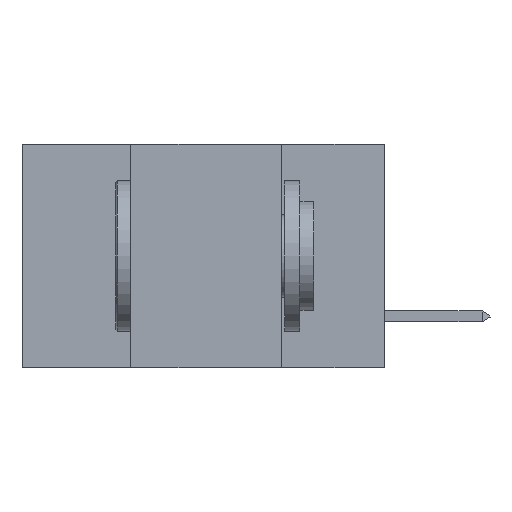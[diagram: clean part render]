
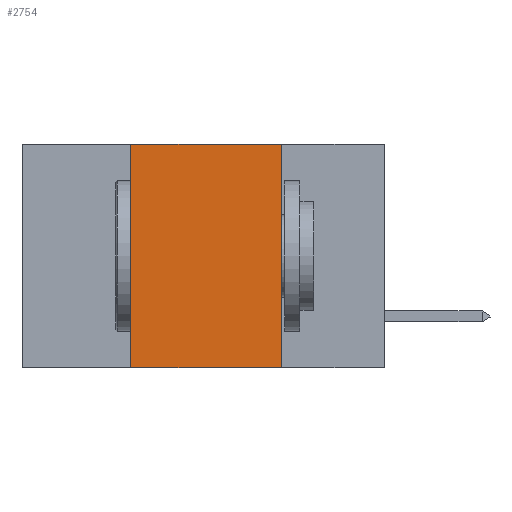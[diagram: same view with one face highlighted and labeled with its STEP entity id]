
A CAD part, left-side view. The second image highlights one B-rep face of the part: STEP entity #2754.
In plain terms, the highlighted planar face has unit normal (-1, 0, 0).
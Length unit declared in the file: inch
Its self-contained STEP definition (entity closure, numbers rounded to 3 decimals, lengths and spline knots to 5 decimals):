
#2 = DIRECTION ( 'NONE',  ( 0., -1., 0. ) ) ;
#82 = DIRECTION ( 'NONE',  ( 0., 0., -1. ) ) ;
#1514 = ORIENTED_EDGE ( 'NONE', *, *, #36094, .F. ) ;
#1586 = VECTOR ( 'NONE', #29866, 39.37008 ) ;
#2420 = VERTEX_POINT ( 'NONE', #3153 ) ;
#2754 = ADVANCED_FACE ( 'NONE', ( #8041 ), #21342, .F. ) ;
#2770 = ORIENTED_EDGE ( 'NONE', *, *, #24472, .F. ) ;
#3153 = CARTESIAN_POINT ( 'NONE',  ( 0., 0.17, -0.37 ) ) ;
#4277 = CARTESIAN_POINT ( 'NONE',  ( 0., 0.17, 0. ) ) ;
#5405 = EDGE_LOOP ( 'NONE', ( #2770, #1514, #38943, #5485 ) ) ;
#5485 = ORIENTED_EDGE ( 'NONE', *, *, #43992, .T. ) ;
#5611 = CARTESIAN_POINT ( 'NONE',  ( 0., 0.17, 0. ) ) ;
#8041 = FACE_OUTER_BOUND ( 'NONE', #5405, .T. ) ;
#8461 = CARTESIAN_POINT ( 'NONE',  ( 0., 0.42, 0. ) ) ;
#8679 = CARTESIAN_POINT ( 'NONE',  ( 0., 0.42, 0. ) ) ;
#11472 = CARTESIAN_POINT ( 'NONE',  ( 0., 0.6, 0. ) ) ;
#12382 = LINE ( 'NONE', #34364, #17732 ) ;
#14783 = VERTEX_POINT ( 'NONE', #8461 ) ;
#17573 = CARTESIAN_POINT ( 'NONE',  ( 0., 0.6, 0. ) ) ;
#17732 = VECTOR ( 'NONE', #2, 39.37008 ) ;
#20066 = LINE ( 'NONE', #5611, #1586 ) ;
#21098 = VERTEX_POINT ( 'NONE', #34168 ) ;
#21342 = PLANE ( 'NONE',  #30249 ) ;
#21563 = EDGE_CURVE ( 'NONE', #21098, #14783, #21848, .T. ) ;
#21848 = LINE ( 'NONE', #8679, #37632 ) ;
#24472 = EDGE_CURVE ( 'NONE', #32337, #2420, #20066, .T. ) ;
#29866 = DIRECTION ( 'NONE',  ( 0., 0., -1. ) ) ;
#30249 = AXIS2_PLACEMENT_3D ( 'NONE', #17573, #38077, #82 ) ;
#32337 = VERTEX_POINT ( 'NONE', #4277 ) ;
#34168 = CARTESIAN_POINT ( 'NONE',  ( 0., 0.42, -0.37 ) ) ;
#34364 = CARTESIAN_POINT ( 'NONE',  ( 0., 0.6, -0.37 ) ) ;
#35889 = VECTOR ( 'NONE', #36667, 39.37008 ) ;
#36094 = EDGE_CURVE ( 'NONE', #14783, #32337, #41891, .T. ) ;
#36667 = DIRECTION ( 'NONE',  ( 0., -1., 0. ) ) ;
#37498 = DIRECTION ( 'NONE',  ( 0., 0., 1. ) ) ;
#37632 = VECTOR ( 'NONE', #37498, 39.37008 ) ;
#38077 = DIRECTION ( 'NONE',  ( 1., 0., 0. ) ) ;
#38943 = ORIENTED_EDGE ( 'NONE', *, *, #21563, .F. ) ;
#41891 = LINE ( 'NONE', #11472, #35889 ) ;
#43992 = EDGE_CURVE ( 'NONE', #21098, #2420, #12382, .T. ) ;
